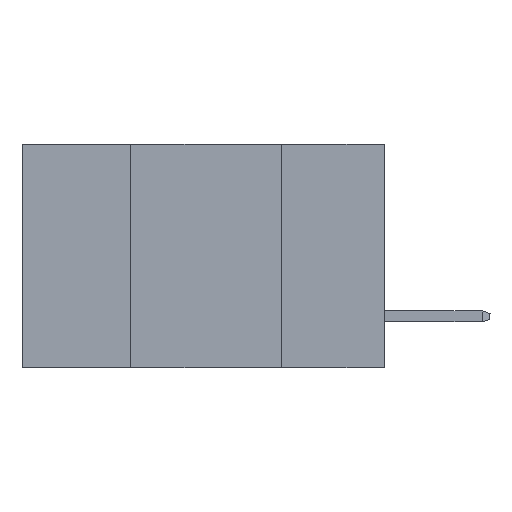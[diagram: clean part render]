
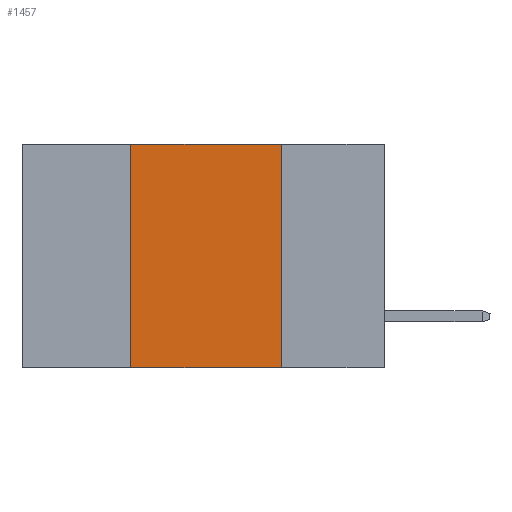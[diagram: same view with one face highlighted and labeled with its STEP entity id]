
A CAD part, left-side view. The second image highlights one B-rep face of the part: STEP entity #1457.
In plain terms, the highlighted planar face has unit normal (-1, 0, 0).
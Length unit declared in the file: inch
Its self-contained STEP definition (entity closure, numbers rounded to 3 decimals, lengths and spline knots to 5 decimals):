
#160 = CARTESIAN_POINT ( 'NONE',  ( 0., 0.6, -0.37 ) ) ;
#370 = VECTOR ( 'NONE', #12667, 39.37008 ) ;
#597 = ORIENTED_EDGE ( 'NONE', *, *, #2059, .F. ) ;
#868 = VECTOR ( 'NONE', #22325, 39.37008 ) ;
#1457 = ADVANCED_FACE ( 'NONE', ( #11737 ), #6278, .F. ) ;
#2059 = EDGE_CURVE ( 'NONE', #16981, #2769, #18359, .T. ) ;
#2769 = VERTEX_POINT ( 'NONE', #4297 ) ;
#3658 = LINE ( 'NONE', #7389, #20036 ) ;
#4293 = DIRECTION ( 'NONE',  ( 1., 0., 0. ) ) ;
#4297 = CARTESIAN_POINT ( 'NONE',  ( 0., 0.42, 0. ) ) ;
#5884 = EDGE_CURVE ( 'NONE', #2769, #21403, #20211, .T. ) ;
#6278 = PLANE ( 'NONE',  #24122 ) ;
#7389 = CARTESIAN_POINT ( 'NONE',  ( 0., 0.17, -0.37 ) ) ;
#10166 = CARTESIAN_POINT ( 'NONE',  ( 0., 0.17, 0. ) ) ;
#10812 = CARTESIAN_POINT ( 'NONE',  ( 0., 0.6, 0. ) ) ;
#11087 = ORIENTED_EDGE ( 'NONE', *, *, #5884, .F. ) ;
#11215 = DIRECTION ( 'NONE',  ( 0., 0., -1. ) ) ;
#11737 = FACE_OUTER_BOUND ( 'NONE', #14786, .T. ) ;
#12022 = CARTESIAN_POINT ( 'NONE',  ( 0., 0.42, -0.37 ) ) ;
#12477 = VERTEX_POINT ( 'NONE', #19332 ) ;
#12667 = DIRECTION ( 'NONE',  ( 0., -1., 0. ) ) ;
#13469 = DIRECTION ( 'NONE',  ( 0., 0., -1. ) ) ;
#14694 = EDGE_CURVE ( 'NONE', #21403, #12477, #3658, .T. ) ;
#14786 = EDGE_LOOP ( 'NONE', ( #22988, #11087, #597, #16653 ) ) ;
#16653 = ORIENTED_EDGE ( 'NONE', *, *, #20812, .T. ) ;
#16981 = VERTEX_POINT ( 'NONE', #12022 ) ;
#17199 = VECTOR ( 'NONE', #18845, 39.37008 ) ;
#18359 = LINE ( 'NONE', #22191, #868 ) ;
#18845 = DIRECTION ( 'NONE',  ( 0., -1., 0. ) ) ;
#19168 = CARTESIAN_POINT ( 'NONE',  ( 0., 0.6, 0. ) ) ;
#19332 = CARTESIAN_POINT ( 'NONE',  ( 0., 0.17, -0.37 ) ) ;
#20036 = VECTOR ( 'NONE', #11215, 39.37008 ) ;
#20211 = LINE ( 'NONE', #10812, #370 ) ;
#20812 = EDGE_CURVE ( 'NONE', #16981, #12477, #20944, .T. ) ;
#20944 = LINE ( 'NONE', #160, #17199 ) ;
#21403 = VERTEX_POINT ( 'NONE', #10166 ) ;
#22191 = CARTESIAN_POINT ( 'NONE',  ( 0., 0.42, -0.37 ) ) ;
#22325 = DIRECTION ( 'NONE',  ( 0., 0., 1. ) ) ;
#22988 = ORIENTED_EDGE ( 'NONE', *, *, #14694, .F. ) ;
#24122 = AXIS2_PLACEMENT_3D ( 'NONE', #19168, #4293, #13469 ) ;
